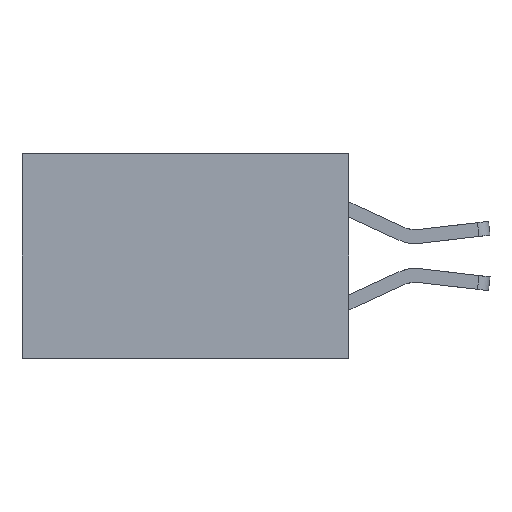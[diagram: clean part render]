
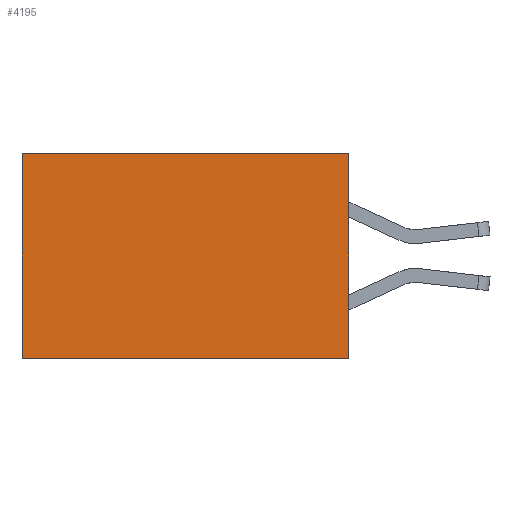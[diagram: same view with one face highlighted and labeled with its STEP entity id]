
A CAD part, left-side view. The second image highlights one B-rep face of the part: STEP entity #4195.
In plain terms, the highlighted planar face has unit normal (-1, 0, 0).
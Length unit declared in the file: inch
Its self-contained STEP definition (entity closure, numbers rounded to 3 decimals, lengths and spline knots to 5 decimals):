
#306 = DIRECTION ( 'NONE',  ( 0., 0., -1. ) ) ;
#320 = CARTESIAN_POINT ( 'NONE',  ( 0.277, 0.59, 0. ) ) ;
#355 = EDGE_LOOP ( 'NONE', ( #2251, #2260, #2289, #2300 ) ) ;
#502 = VERTEX_POINT ( 'NONE', #3955 ) ;
#713 = CARTESIAN_POINT ( 'NONE',  ( 0.277, 0., -0.37 ) ) ;
#758 = DIRECTION ( 'NONE',  ( 0., 1., 0. ) ) ;
#811 = FACE_OUTER_BOUND ( 'NONE', #355, .T. ) ;
#1027 = LINE ( 'NONE', #3926, #7573 ) ;
#2251 = ORIENTED_EDGE ( 'NONE', *, *, #6280, .T. ) ;
#2260 = ORIENTED_EDGE ( 'NONE', *, *, #5940, .F. ) ;
#2289 = ORIENTED_EDGE ( 'NONE', *, *, #5154, .F. ) ;
#2300 = ORIENTED_EDGE ( 'NONE', *, *, #7515, .T. ) ;
#2463 = VERTEX_POINT ( 'NONE', #713 ) ;
#2629 = DIRECTION ( 'NONE',  ( 0., 1., 0. ) ) ;
#2667 = CARTESIAN_POINT ( 'NONE',  ( 0.277, 0., 0. ) ) ;
#3200 = DIRECTION ( 'NONE',  ( 0., 0., -1. ) ) ;
#3565 = LINE ( 'NONE', #5726, #7918 ) ;
#3849 = CARTESIAN_POINT ( 'NONE',  ( 0.277, 0., 0. ) ) ;
#3926 = CARTESIAN_POINT ( 'NONE',  ( 0.277, 0., -0.37 ) ) ;
#3929 = CARTESIAN_POINT ( 'NONE',  ( 0.277, 0.59, -0.37 ) ) ;
#3955 = CARTESIAN_POINT ( 'NONE',  ( 0.277, 0.59, -0.37 ) ) ;
#4195 = ADVANCED_FACE ( 'NONE', ( #811 ), #7210, .F. ) ;
#4247 = LINE ( 'NONE', #2667, #4443 ) ;
#4278 = DIRECTION ( 'NONE',  ( 0., 0., -1. ) ) ;
#4342 = AXIS2_PLACEMENT_3D ( 'NONE', #5985, #5494, #306 ) ;
#4443 = VECTOR ( 'NONE', #2629, 39.37008 ) ;
#4739 = LINE ( 'NONE', #3929, #7462 ) ;
#5154 = EDGE_CURVE ( 'NONE', #7354, #2463, #1027, .T. ) ;
#5494 = DIRECTION ( 'NONE',  ( 1., 0., 0. ) ) ;
#5726 = CARTESIAN_POINT ( 'NONE',  ( 0.277, 0., -0.37 ) ) ;
#5940 = EDGE_CURVE ( 'NONE', #2463, #502, #3565, .T. ) ;
#5985 = CARTESIAN_POINT ( 'NONE',  ( 0.277, 0., -0.37 ) ) ;
#6280 = EDGE_CURVE ( 'NONE', #6398, #502, #4739, .T. ) ;
#6398 = VERTEX_POINT ( 'NONE', #320 ) ;
#7210 = PLANE ( 'NONE',  #4342 ) ;
#7354 = VERTEX_POINT ( 'NONE', #3849 ) ;
#7462 = VECTOR ( 'NONE', #3200, 39.37008 ) ;
#7515 = EDGE_CURVE ( 'NONE', #7354, #6398, #4247, .T. ) ;
#7573 = VECTOR ( 'NONE', #4278, 39.37008 ) ;
#7918 = VECTOR ( 'NONE', #758, 39.37008 ) ;
